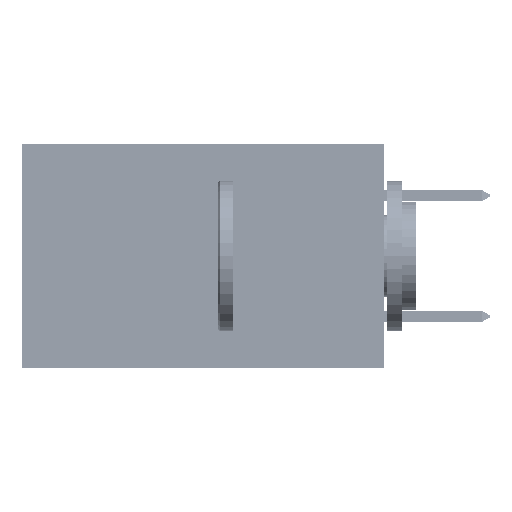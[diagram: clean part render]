
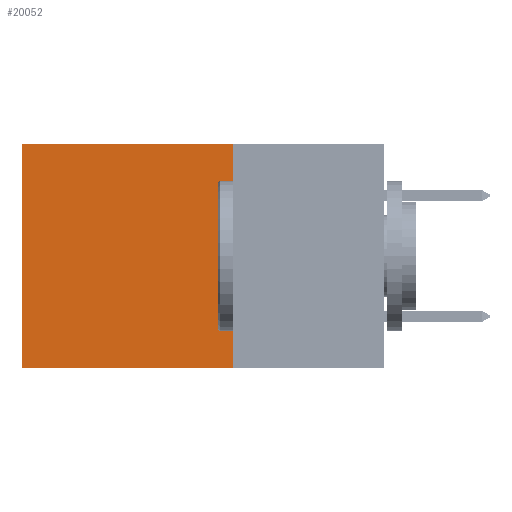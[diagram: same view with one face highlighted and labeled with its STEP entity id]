
A CAD part, left-side view. The second image highlights one B-rep face of the part: STEP entity #20052.
In plain terms, the highlighted planar face has unit normal (-1, 0, 0).
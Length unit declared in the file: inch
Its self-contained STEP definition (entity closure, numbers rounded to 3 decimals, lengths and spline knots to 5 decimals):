
#911 = DIRECTION ( 'NONE',  ( 0., 1., 0. ) ) ;
#2174 = DIRECTION ( 'NONE',  ( 0., 0., -1. ) ) ;
#3101 = DIRECTION ( 'NONE',  ( 1., 0., 0. ) ) ;
#3539 = LINE ( 'NONE', #15129, #4649 ) ;
#4649 = VECTOR ( 'NONE', #911, 39.37008 ) ;
#5437 = EDGE_CURVE ( 'NONE', #15704, #27529, #43661, .T. ) ;
#7096 = DIRECTION ( 'NONE',  ( 0., 1., 0. ) ) ;
#7542 = VECTOR ( 'NONE', #18007, 39.37008 ) ;
#8433 = LINE ( 'NONE', #44773, #43849 ) ;
#10050 = EDGE_LOOP ( 'NONE', ( #37595, #18482, #38096, #34008 ) ) ;
#10086 = EDGE_CURVE ( 'NONE', #15704, #15159, #8433, .T. ) ;
#15129 = CARTESIAN_POINT ( 'NONE',  ( 0.2875, 0.25, -0.37 ) ) ;
#15159 = VERTEX_POINT ( 'NONE', #37997 ) ;
#15704 = VERTEX_POINT ( 'NONE', #27279 ) ;
#18007 = DIRECTION ( 'NONE',  ( 0., 0., -1. ) ) ;
#18482 = ORIENTED_EDGE ( 'NONE', *, *, #35909, .F. ) ;
#20052 = ADVANCED_FACE ( 'NONE', ( #22086 ), #20757, .F. ) ;
#20757 = PLANE ( 'NONE',  #32104 ) ;
#22086 = FACE_OUTER_BOUND ( 'NONE', #10050, .T. ) ;
#22860 = CARTESIAN_POINT ( 'NONE',  ( 0.2875, 0.6, -0.37 ) ) ;
#23352 = CARTESIAN_POINT ( 'NONE',  ( 0.2875, 0.25, 0. ) ) ;
#25138 = LINE ( 'NONE', #28393, #7542 ) ;
#26686 = EDGE_CURVE ( 'NONE', #15159, #44482, #25138, .T. ) ;
#27279 = CARTESIAN_POINT ( 'NONE',  ( 0.2875, 0.25, 0. ) ) ;
#27529 = VERTEX_POINT ( 'NONE', #40016 ) ;
#27640 = DIRECTION ( 'NONE',  ( 0., 0., -1. ) ) ;
#28393 = CARTESIAN_POINT ( 'NONE',  ( 0.2875, 0.6, 0. ) ) ;
#32104 = AXIS2_PLACEMENT_3D ( 'NONE', #44386, #3101, #27640 ) ;
#34008 = ORIENTED_EDGE ( 'NONE', *, *, #10086, .T. ) ;
#35881 = VECTOR ( 'NONE', #2174, 39.37008 ) ;
#35909 = EDGE_CURVE ( 'NONE', #27529, #44482, #3539, .T. ) ;
#37595 = ORIENTED_EDGE ( 'NONE', *, *, #26686, .T. ) ;
#37997 = CARTESIAN_POINT ( 'NONE',  ( 0.2875, 0.6, 0. ) ) ;
#38096 = ORIENTED_EDGE ( 'NONE', *, *, #5437, .F. ) ;
#40016 = CARTESIAN_POINT ( 'NONE',  ( 0.2875, 0.25, -0.37 ) ) ;
#43661 = LINE ( 'NONE', #23352, #35881 ) ;
#43849 = VECTOR ( 'NONE', #7096, 39.37008 ) ;
#44386 = CARTESIAN_POINT ( 'NONE',  ( 0.2875, 0.25, 0. ) ) ;
#44482 = VERTEX_POINT ( 'NONE', #22860 ) ;
#44773 = CARTESIAN_POINT ( 'NONE',  ( 0.2875, 0.25, 0. ) ) ;
